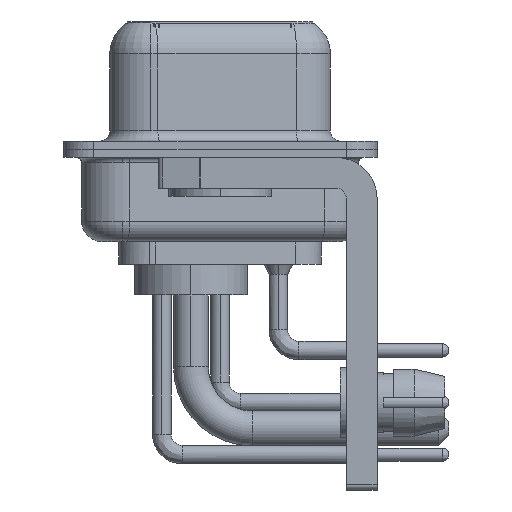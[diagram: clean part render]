
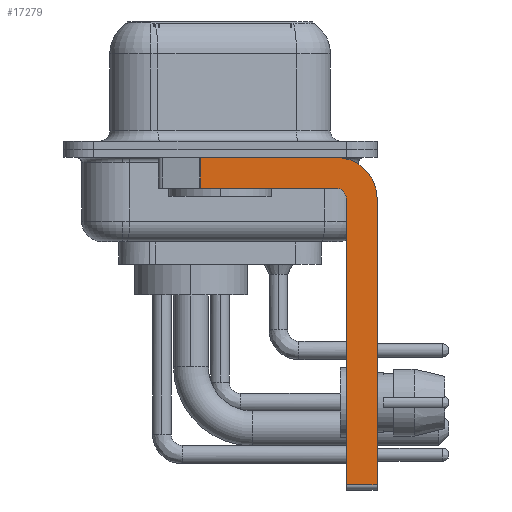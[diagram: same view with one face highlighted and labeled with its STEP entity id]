
A CAD part, left-side view. The second image highlights one B-rep face of the part: STEP entity #17279.
In plain terms, the highlighted planar face has unit normal (-1, 0, 0).
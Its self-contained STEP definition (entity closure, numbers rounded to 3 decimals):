
#51 = VERTEX_POINT ( 'NONE', #28266 ) ;
#123 = VECTOR ( 'NONE', #12548, 1000. ) ;
#244 = DIRECTION ( 'NONE',  ( 0., 1., 0. ) ) ;
#1341 = DIRECTION ( 'NONE',  ( 0., 0., -1. ) ) ;
#2976 = LINE ( 'NONE', #12477, #12465 ) ;
#3078 = VERTEX_POINT ( 'NONE', #10888 ) ;
#4433 = LINE ( 'NONE', #14557, #13992 ) ;
#4553 = CARTESIAN_POINT ( 'NONE',  ( -2.9, -7.65, -2.4 ) ) ;
#5121 = AXIS2_PLACEMENT_3D ( 'NONE', #19924, #8056, #20235 ) ;
#5431 = DIRECTION ( 'NONE',  ( 0., 0., -1. ) ) ;
#6335 = ORIENTED_EDGE ( 'NONE', *, *, #15677, .F. ) ;
#6567 = CIRCLE ( 'NONE', #10190, 2. ) ;
#7168 = CIRCLE ( 'NONE', #5121, 0.5 ) ;
#7439 = VECTOR ( 'NONE', #29113, 1000. ) ;
#7633 = VERTEX_POINT ( 'NONE', #12778 ) ;
#8022 = LINE ( 'NONE', #10456, #123 ) ;
#8039 = EDGE_CURVE ( 'NONE', #30377, #27487, #15732, .T. ) ;
#8056 = DIRECTION ( 'NONE',  ( -1., 0., 0. ) ) ;
#8160 = DIRECTION ( 'NONE',  ( 1., 0., 0. ) ) ;
#10190 = AXIS2_PLACEMENT_3D ( 'NONE', #22583, #8160, #5431 ) ;
#10456 = CARTESIAN_POINT ( 'NONE',  ( -2.9, -6.15, -16.6 ) ) ;
#10888 = CARTESIAN_POINT ( 'NONE',  ( -2.9, -5.65, -0.4 ) ) ;
#10967 = ORIENTED_EDGE ( 'NONE', *, *, #23802, .F. ) ;
#11175 = EDGE_LOOP ( 'NONE', ( #14134, #15044, #28089, #10967, #19841, #23003, #6335, #26599 ) ) ;
#12286 = VECTOR ( 'NONE', #244, 1000. ) ;
#12465 = VECTOR ( 'NONE', #15183, 1000. ) ;
#12477 = CARTESIAN_POINT ( 'NONE',  ( -2.9, 0.978, -1.9 ) ) ;
#12548 = DIRECTION ( 'NONE',  ( 0., 0., 1. ) ) ;
#12778 = CARTESIAN_POINT ( 'NONE',  ( -2.9, 0.978, -1.9 ) ) ;
#13517 = CARTESIAN_POINT ( 'NONE',  ( -2.9, -6.15, -2.4 ) ) ;
#13761 = EDGE_CURVE ( 'NONE', #30059, #3078, #4433, .T. ) ;
#13848 = CARTESIAN_POINT ( 'NONE',  ( -2.9, 0.978, -0.4 ) ) ;
#13992 = VECTOR ( 'NONE', #21757, 1000. ) ;
#14134 = ORIENTED_EDGE ( 'NONE', *, *, #13761, .F. ) ;
#14557 = CARTESIAN_POINT ( 'NONE',  ( -2.9, 3., -0.4 ) ) ;
#15044 = ORIENTED_EDGE ( 'NONE', *, *, #26400, .T. ) ;
#15183 = DIRECTION ( 'NONE',  ( 0., 0., -1. ) ) ;
#15677 = EDGE_CURVE ( 'NONE', #51, #27487, #16759, .T. ) ;
#15732 = LINE ( 'NONE', #17971, #21937 ) ;
#16315 = CARTESIAN_POINT ( 'NONE',  ( -2.9, -5.65, -1.9 ) ) ;
#16759 = LINE ( 'NONE', #4553, #7439 ) ;
#17279 = ADVANCED_FACE ( 'NONE', ( #31183 ), #25871, .F. ) ;
#17971 = CARTESIAN_POINT ( 'NONE',  ( -2.9, -5.65, -16.35 ) ) ;
#18661 = CARTESIAN_POINT ( 'NONE',  ( -2.9, -5.65, -2.4 ) ) ;
#19841 = ORIENTED_EDGE ( 'NONE', *, *, #25489, .F. ) ;
#19919 = CARTESIAN_POINT ( 'NONE',  ( -2.9, -6.15, -16.35 ) ) ;
#19924 = CARTESIAN_POINT ( 'NONE',  ( -2.9, -5.65, -2.4 ) ) ;
#20235 = DIRECTION ( 'NONE',  ( 0., 0., 1. ) ) ;
#20889 = DIRECTION ( 'NONE',  ( 1., 0., 0. ) ) ;
#20926 = EDGE_CURVE ( 'NONE', #3078, #51, #6567, .T. ) ;
#21419 = CARTESIAN_POINT ( 'NONE',  ( -2.9, -7.65, -16.35 ) ) ;
#21757 = DIRECTION ( 'NONE',  ( 0., -1., 0. ) ) ;
#21867 = VERTEX_POINT ( 'NONE', #29042 ) ;
#21937 = VECTOR ( 'NONE', #27754, 1000. ) ;
#22583 = CARTESIAN_POINT ( 'NONE',  ( -2.9, -5.65, -2.4 ) ) ;
#22974 = EDGE_CURVE ( 'NONE', #21867, #7633, #30756, .T. ) ;
#23003 = ORIENTED_EDGE ( 'NONE', *, *, #8039, .T. ) ;
#23802 = EDGE_CURVE ( 'NONE', #30481, #21867, #7168, .T. ) ;
#25489 = EDGE_CURVE ( 'NONE', #30377, #30481, #8022, .T. ) ;
#25871 = PLANE ( 'NONE',  #31523 ) ;
#26400 = EDGE_CURVE ( 'NONE', #30059, #7633, #2976, .T. ) ;
#26599 = ORIENTED_EDGE ( 'NONE', *, *, #20926, .F. ) ;
#27487 = VERTEX_POINT ( 'NONE', #21419 ) ;
#27754 = DIRECTION ( 'NONE',  ( 0., -1., 0. ) ) ;
#28089 = ORIENTED_EDGE ( 'NONE', *, *, #22974, .F. ) ;
#28266 = CARTESIAN_POINT ( 'NONE',  ( -2.9, -7.65, -2.4 ) ) ;
#29042 = CARTESIAN_POINT ( 'NONE',  ( -2.9, -5.65, -1.9 ) ) ;
#29113 = DIRECTION ( 'NONE',  ( 0., 0., -1. ) ) ;
#30059 = VERTEX_POINT ( 'NONE', #13848 ) ;
#30377 = VERTEX_POINT ( 'NONE', #19919 ) ;
#30481 = VERTEX_POINT ( 'NONE', #13517 ) ;
#30756 = LINE ( 'NONE', #16315, #12286 ) ;
#31183 = FACE_OUTER_BOUND ( 'NONE', #11175, .T. ) ;
#31523 = AXIS2_PLACEMENT_3D ( 'NONE', #18661, #20889, #1341 ) ;
